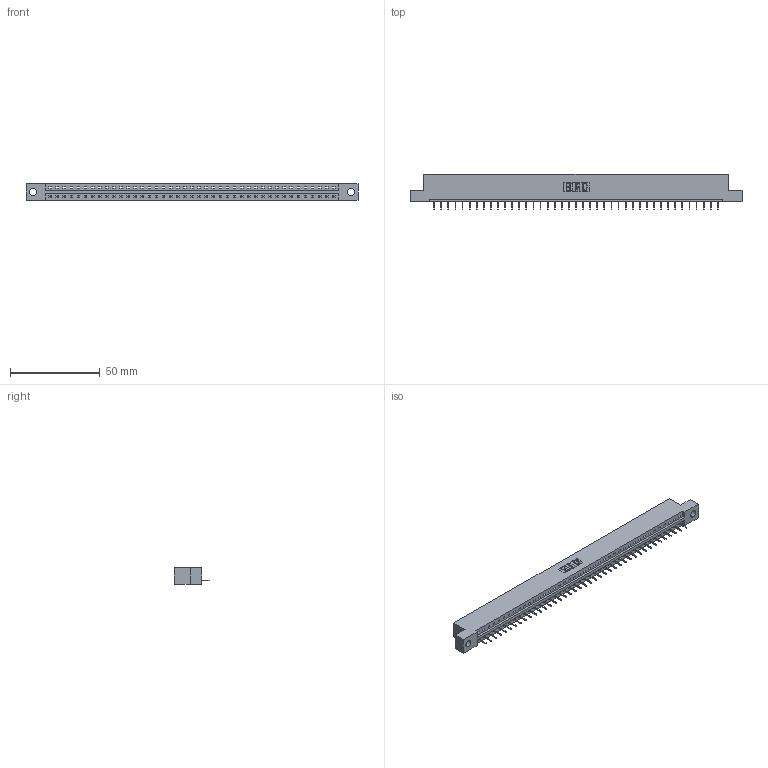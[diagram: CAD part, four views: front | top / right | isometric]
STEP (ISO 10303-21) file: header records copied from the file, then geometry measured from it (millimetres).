
FILE_DESCRIPTION (( 'STEP AP203' ), '1' );
FILE_NAME ('387-041-524-104.STEP', '2018-09-19T18:02:23', ( '' ), ( '' ), 'SwSTEP 2.0', 'SolidWorks 2016', '' );
FILE_SCHEMA (( 'CONFIG_CONTROL_DESIGN' ));
Length unit declared in the file: inch
Products named in the file (3): 337 Part_Flush Mounting Lugs - 0.156 Dia-TH; 345-292-001_345-293-124; 387-041-524-104
Assembly tree (42 placements, depth 2):
  387-041-524-104
    337 Part_Flush Mounting Lugs - 0.156 Dia-TH
    345-292-001_345-293-124  x41
Bounding box: 185.47 x 19.69 x 9.4 mm (x, y, z)
Volume: 19014.2 mm3; surface area: 18868.6 mm2
Topology: 42 solids, 42 shells, 2820 faces, 8183 edges, 5290 vertices
Faces by surface type: plane 2202, cylinder 618
Entity records: 30683 total; most frequent: CARTESIAN_POINT 5349, ORIENTED_EDGE 5326, DIRECTION 4505, EDGE_CURVE 2663, LINE 2539, VECTOR 2539, VERTEX_POINT 1770, AXIS2_PLACEMENT_3D 983
